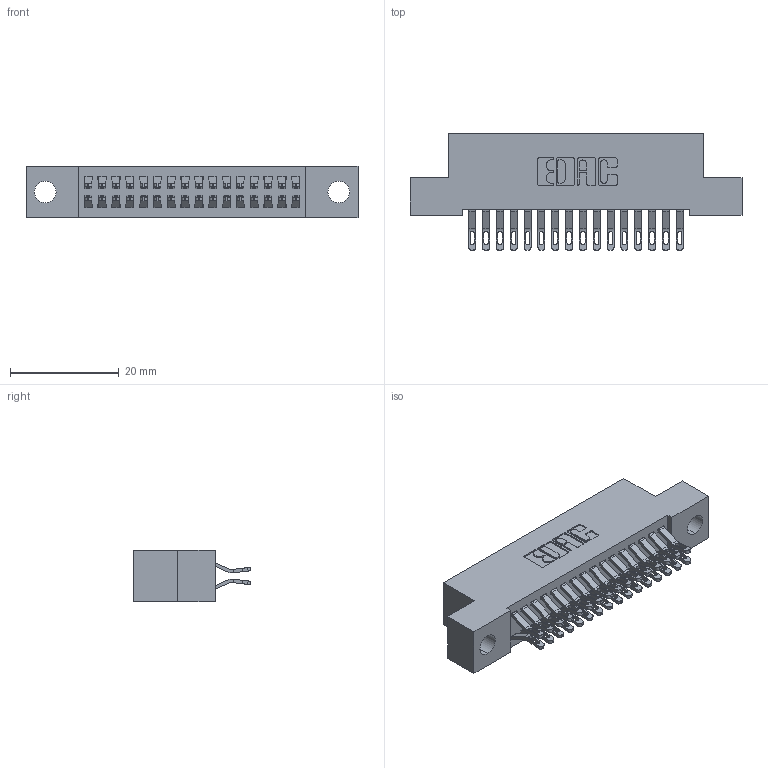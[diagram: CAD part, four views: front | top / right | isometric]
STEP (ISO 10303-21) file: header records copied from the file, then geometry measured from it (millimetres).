
FILE_DESCRIPTION (( 'STEP AP203' ), '1' );
FILE_NAME ('392-032-555-204.STEP', '2018-08-16T00:17:51', ( '' ), ( '' ), 'SwSTEP 2.0', 'SolidWorks 2016', '' );
FILE_SCHEMA (( 'CONFIG_CONTROL_DESIGN' ));
Length unit declared in the file: inch
Products named in the file (3): 342 Part_.156 TH; 345-292-001_555 Tail; 392-032-555-204
Assembly tree (33 placements, depth 2):
  392-032-555-204
    342 Part_.156 TH
    345-292-001_555 Tail  x32
Bounding box: 60.96 x 21.47 x 9.4 mm (x, y, z)
Volume: 5356.1 mm3; surface area: 8211.5 mm2
Topology: 33 solids, 33 shells, 1966 faces, 6155 edges, 4102 vertices
Faces by surface type: plane 1154, cylinder 812
Entity records: 13853 total; most frequent: CARTESIAN_POINT 2360, ORIENTED_EDGE 2266, DIRECTION 2033, EDGE_CURVE 1133, LINE 985, VECTOR 985, VERTEX_POINT 754, AXIS2_PLACEMENT_3D 524
